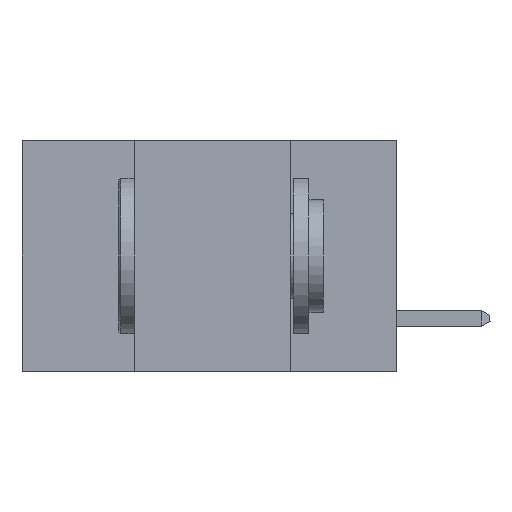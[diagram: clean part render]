
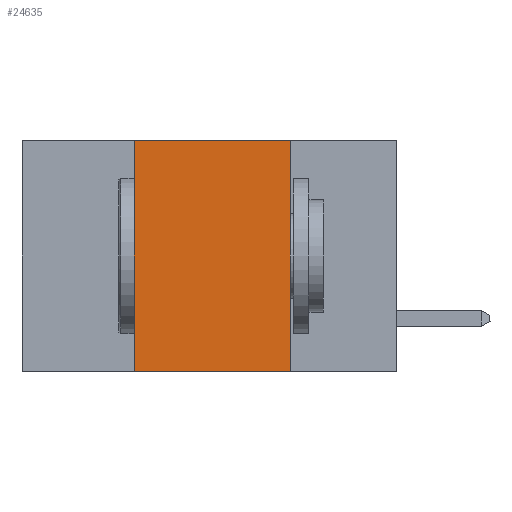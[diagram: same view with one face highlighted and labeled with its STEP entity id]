
A CAD part, left-side view. The second image highlights one B-rep face of the part: STEP entity #24635.
In plain terms, the highlighted planar face has unit normal (-1, 0, 0).
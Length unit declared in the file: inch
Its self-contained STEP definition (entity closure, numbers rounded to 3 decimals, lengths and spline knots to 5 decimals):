
#201 = ORIENTED_EDGE ( 'NONE', *, *, #902, .F. ) ;
#223 = VERTEX_POINT ( 'NONE', #8865 ) ;
#902 = EDGE_CURVE ( 'NONE', #12542, #223, #4024, .T. ) ;
#937 = PLANE ( 'NONE',  #18482 ) ;
#2081 = VECTOR ( 'NONE', #7734, 39.37008 ) ;
#3189 = CARTESIAN_POINT ( 'NONE',  ( 0., 0.6, 0. ) ) ;
#3287 = DIRECTION ( 'NONE',  ( 0., 0., 1. ) ) ;
#3933 = LINE ( 'NONE', #19682, #26424 ) ;
#4024 = LINE ( 'NONE', #20641, #25860 ) ;
#5403 = DIRECTION ( 'NONE',  ( 1., 0., 0. ) ) ;
#5816 = VECTOR ( 'NONE', #21730, 39.37008 ) ;
#7734 = DIRECTION ( 'NONE',  ( 0., -1., 0. ) ) ;
#7754 = CARTESIAN_POINT ( 'NONE',  ( 0., 0.17, 0. ) ) ;
#7825 = CARTESIAN_POINT ( 'NONE',  ( 0., 0.6, -0.37 ) ) ;
#8865 = CARTESIAN_POINT ( 'NONE',  ( 0., 0.42, 0. ) ) ;
#10123 = ORIENTED_EDGE ( 'NONE', *, *, #17638, .T. ) ;
#11633 = LINE ( 'NONE', #19531, #5816 ) ;
#11635 = VERTEX_POINT ( 'NONE', #13307 ) ;
#11925 = CARTESIAN_POINT ( 'NONE',  ( 0., 0.42, -0.37 ) ) ;
#12251 = EDGE_CURVE ( 'NONE', #223, #24023, #3933, .T. ) ;
#12542 = VERTEX_POINT ( 'NONE', #11925 ) ;
#13307 = CARTESIAN_POINT ( 'NONE',  ( 0., 0.17, -0.37 ) ) ;
#13736 = LINE ( 'NONE', #7825, #2081 ) ;
#16001 = ORIENTED_EDGE ( 'NONE', *, *, #12251, .F. ) ;
#17638 = EDGE_CURVE ( 'NONE', #12542, #11635, #13736, .T. ) ;
#18482 = AXIS2_PLACEMENT_3D ( 'NONE', #3189, #5403, #20713 ) ;
#18554 = EDGE_CURVE ( 'NONE', #24023, #11635, #11633, .T. ) ;
#19531 = CARTESIAN_POINT ( 'NONE',  ( 0., 0.17, 0. ) ) ;
#19682 = CARTESIAN_POINT ( 'NONE',  ( 0., 0.6, 0. ) ) ;
#20641 = CARTESIAN_POINT ( 'NONE',  ( 0., 0.42, 0. ) ) ;
#20713 = DIRECTION ( 'NONE',  ( 0., 0., -1. ) ) ;
#20868 = EDGE_LOOP ( 'NONE', ( #27930, #16001, #201, #10123 ) ) ;
#21730 = DIRECTION ( 'NONE',  ( 0., 0., -1. ) ) ;
#21876 = DIRECTION ( 'NONE',  ( 0., -1., 0. ) ) ;
#24023 = VERTEX_POINT ( 'NONE', #7754 ) ;
#24635 = ADVANCED_FACE ( 'NONE', ( #26266 ), #937, .F. ) ;
#25860 = VECTOR ( 'NONE', #3287, 39.37008 ) ;
#26266 = FACE_OUTER_BOUND ( 'NONE', #20868, .T. ) ;
#26424 = VECTOR ( 'NONE', #21876, 39.37008 ) ;
#27930 = ORIENTED_EDGE ( 'NONE', *, *, #18554, .F. ) ;
